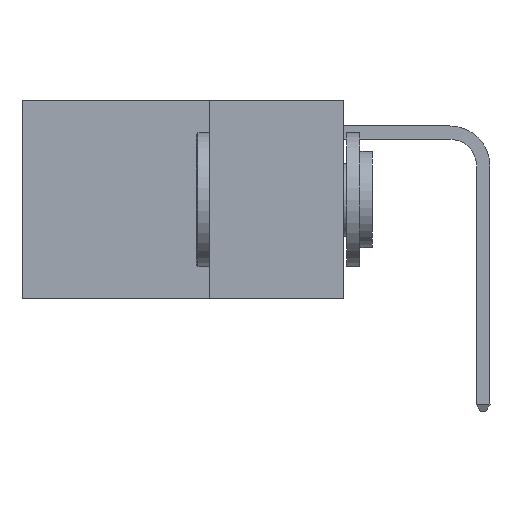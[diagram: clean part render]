
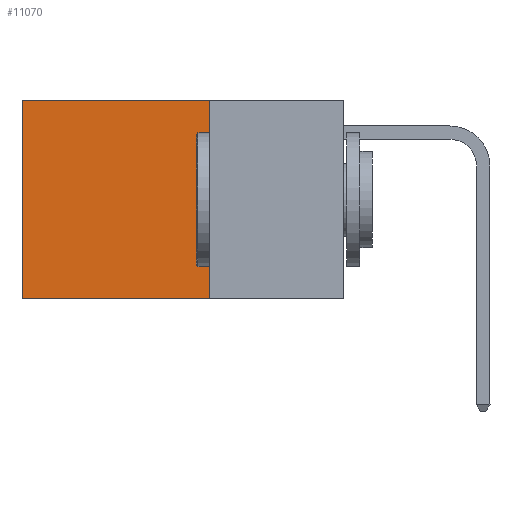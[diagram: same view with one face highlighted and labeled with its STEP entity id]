
A CAD part, left-side view. The second image highlights one B-rep face of the part: STEP entity #11070.
In plain terms, the highlighted planar face has unit normal (-1, 0, 0).
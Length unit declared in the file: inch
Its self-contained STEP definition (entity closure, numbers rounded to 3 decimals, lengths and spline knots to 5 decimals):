
#1498 = VERTEX_POINT ( 'NONE', #10695 ) ;
#1769 = VERTEX_POINT ( 'NONE', #3616 ) ;
#2120 = CARTESIAN_POINT ( 'NONE',  ( 0.2625, 0.25, -0.37 ) ) ;
#2247 = CARTESIAN_POINT ( 'NONE',  ( 0.2625, 0.6, 0. ) ) ;
#2371 = ORIENTED_EDGE ( 'NONE', *, *, #5090, .T. ) ;
#2508 = CARTESIAN_POINT ( 'NONE',  ( 0.2625, 0.25, 0. ) ) ;
#3466 = CARTESIAN_POINT ( 'NONE',  ( 0.2625, 0.25, 0. ) ) ;
#3616 = CARTESIAN_POINT ( 'NONE',  ( 0.2625, 0.25, -0.37 ) ) ;
#4053 = AXIS2_PLACEMENT_3D ( 'NONE', #3466, #11076, #4540 ) ;
#4178 = DIRECTION ( 'NONE',  ( 0., 1., 0. ) ) ;
#4450 = ORIENTED_EDGE ( 'NONE', *, *, #6604, .F. ) ;
#4540 = DIRECTION ( 'NONE',  ( 0., 0., -1. ) ) ;
#4663 = CARTESIAN_POINT ( 'NONE',  ( 0.2625, 0.25, 0. ) ) ;
#5079 = LINE ( 'NONE', #2120, #13063 ) ;
#5090 = EDGE_CURVE ( 'NONE', #1498, #8650, #12293, .T. ) ;
#5258 = FACE_OUTER_BOUND ( 'NONE', #10631, .T. ) ;
#5339 = LINE ( 'NONE', #2508, #13309 ) ;
#6232 = ORIENTED_EDGE ( 'NONE', *, *, #14062, .F. ) ;
#6604 = EDGE_CURVE ( 'NONE', #1769, #9137, #5079, .T. ) ;
#7488 = LINE ( 'NONE', #2247, #10011 ) ;
#7984 = DIRECTION ( 'NONE',  ( 0., 0., -1. ) ) ;
#8650 = VERTEX_POINT ( 'NONE', #14027 ) ;
#8845 = DIRECTION ( 'NONE',  ( 0., 0., -1. ) ) ;
#9137 = VERTEX_POINT ( 'NONE', #11765 ) ;
#9447 = VECTOR ( 'NONE', #4178, 39.37008 ) ;
#9806 = DIRECTION ( 'NONE',  ( 0., 1., 0. ) ) ;
#10001 = PLANE ( 'NONE',  #4053 ) ;
#10011 = VECTOR ( 'NONE', #8845, 39.37008 ) ;
#10631 = EDGE_LOOP ( 'NONE', ( #13355, #4450, #6232, #2371 ) ) ;
#10695 = CARTESIAN_POINT ( 'NONE',  ( 0.2625, 0.25, 0. ) ) ;
#11070 = ADVANCED_FACE ( 'NONE', ( #5258 ), #10001, .F. ) ;
#11076 = DIRECTION ( 'NONE',  ( 1., 0., 0. ) ) ;
#11765 = CARTESIAN_POINT ( 'NONE',  ( 0.2625, 0.6, -0.37 ) ) ;
#12293 = LINE ( 'NONE', #4663, #9447 ) ;
#12656 = EDGE_CURVE ( 'NONE', #8650, #9137, #7488, .T. ) ;
#13063 = VECTOR ( 'NONE', #9806, 39.37008 ) ;
#13309 = VECTOR ( 'NONE', #7984, 39.37008 ) ;
#13355 = ORIENTED_EDGE ( 'NONE', *, *, #12656, .T. ) ;
#14027 = CARTESIAN_POINT ( 'NONE',  ( 0.2625, 0.6, 0. ) ) ;
#14062 = EDGE_CURVE ( 'NONE', #1498, #1769, #5339, .T. ) ;
